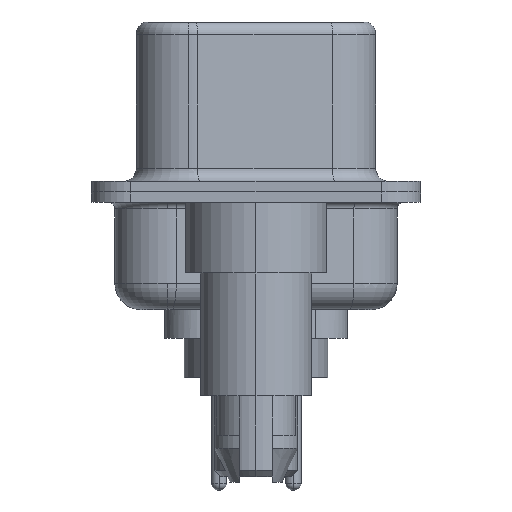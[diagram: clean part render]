
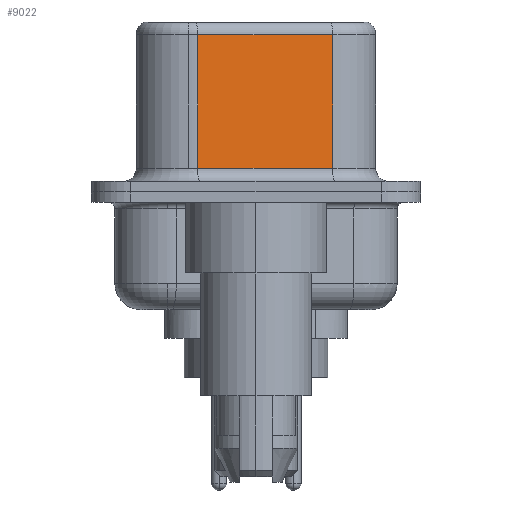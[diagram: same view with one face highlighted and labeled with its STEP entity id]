
A CAD part, left-side view. The second image highlights one B-rep face of the part: STEP entity #9022.
In plain terms, the highlighted planar face has unit normal (-0.985, -0.174, 0).
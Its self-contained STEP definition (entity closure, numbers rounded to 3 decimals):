
#61 = AXIS2_PLACEMENT_3D ( 'NONE', #14055, #8990, #1162 ) ;
#686 = VERTEX_POINT ( 'NONE', #12565 ) ;
#770 = ORIENTED_EDGE ( 'NONE', *, *, #6237, .T. ) ;
#1162 = DIRECTION ( 'NONE',  ( -0.174, 0.985, 0. ) ) ;
#1353 = VECTOR ( 'NONE', #5832, 1000. ) ;
#2015 = CARTESIAN_POINT ( 'NONE',  ( 4.565, -2.927, 0.9 ) ) ;
#2038 = LINE ( 'NONE', #7081, #12045 ) ;
#2088 = CARTESIAN_POINT ( 'NONE',  ( 4.565, -2.927, 0.9 ) ) ;
#2113 = VERTEX_POINT ( 'NONE', #4117 ) ;
#4117 = CARTESIAN_POINT ( 'NONE',  ( 3.655, 2.233, 6.02 ) ) ;
#5103 = ORIENTED_EDGE ( 'NONE', *, *, #14586, .T. ) ;
#5770 = CARTESIAN_POINT ( 'NONE',  ( 3.655, 2.233, 6.52 ) ) ;
#5832 = DIRECTION ( 'NONE',  ( 0., 0., -1. ) ) ;
#6165 = EDGE_CURVE ( 'NONE', #686, #13485, #11753, .T. ) ;
#6171 = VECTOR ( 'NONE', #8593, 1000. ) ;
#6237 = EDGE_CURVE ( 'NONE', #13263, #13485, #9765, .T. ) ;
#7081 = CARTESIAN_POINT ( 'NONE',  ( 4.565, -2.927, 6.02 ) ) ;
#7786 = EDGE_LOOP ( 'NONE', ( #13271, #13469, #5103, #770 ) ) ;
#8415 = DIRECTION ( 'NONE',  ( 0., 0., -1. ) ) ;
#8442 = LINE ( 'NONE', #5770, #14810 ) ;
#8593 = DIRECTION ( 'NONE',  ( 0.174, -0.985, 0. ) ) ;
#8862 = EDGE_CURVE ( 'NONE', #686, #2113, #2038, .T. ) ;
#8990 = DIRECTION ( 'NONE',  ( 0.985, 0.174, 0. ) ) ;
#9022 = ADVANCED_FACE ( 'NONE', ( #9657 ), #16473, .F. ) ;
#9564 = CARTESIAN_POINT ( 'NONE',  ( 3.655, 2.233, 0.9 ) ) ;
#9657 = FACE_OUTER_BOUND ( 'NONE', #7786, .T. ) ;
#9765 = LINE ( 'NONE', #2088, #6171 ) ;
#11753 = LINE ( 'NONE', #12342, #1353 ) ;
#12045 = VECTOR ( 'NONE', #12317, 1000. ) ;
#12317 = DIRECTION ( 'NONE',  ( -0.174, 0.985, 0. ) ) ;
#12342 = CARTESIAN_POINT ( 'NONE',  ( 4.565, -2.927, 6.52 ) ) ;
#12565 = CARTESIAN_POINT ( 'NONE',  ( 4.565, -2.927, 6.02 ) ) ;
#13263 = VERTEX_POINT ( 'NONE', #9564 ) ;
#13271 = ORIENTED_EDGE ( 'NONE', *, *, #6165, .F. ) ;
#13469 = ORIENTED_EDGE ( 'NONE', *, *, #8862, .T. ) ;
#13485 = VERTEX_POINT ( 'NONE', #2015 ) ;
#14055 = CARTESIAN_POINT ( 'NONE',  ( 4.565, -2.927, 6.52 ) ) ;
#14586 = EDGE_CURVE ( 'NONE', #2113, #13263, #8442, .T. ) ;
#14810 = VECTOR ( 'NONE', #8415, 1000. ) ;
#16473 = PLANE ( 'NONE',  #61 ) ;
